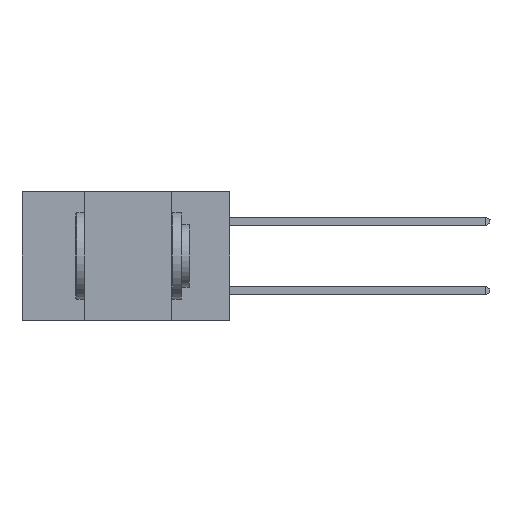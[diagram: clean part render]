
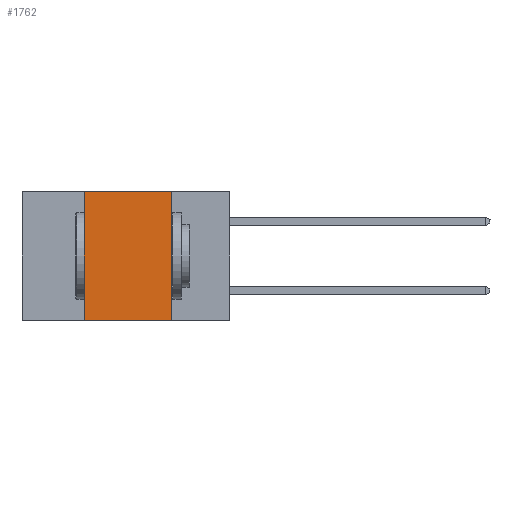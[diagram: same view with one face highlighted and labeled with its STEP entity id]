
A CAD part, left-side view. The second image highlights one B-rep face of the part: STEP entity #1762.
In plain terms, the highlighted planar face has unit normal (-1, 0, 0).
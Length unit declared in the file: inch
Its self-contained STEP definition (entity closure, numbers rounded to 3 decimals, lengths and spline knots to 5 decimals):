
#173 = CARTESIAN_POINT ( 'NONE',  ( 0., 0.6, 0. ) ) ;
#1762 = ADVANCED_FACE ( 'NONE', ( #4417 ), #4195, .F. ) ;
#1838 = CARTESIAN_POINT ( 'NONE',  ( 0., 0.42, -0.37 ) ) ;
#1903 = VECTOR ( 'NONE', #13524, 39.37008 ) ;
#2373 = EDGE_LOOP ( 'NONE', ( #3141, #16533, #15461, #11650 ) ) ;
#2623 = VECTOR ( 'NONE', #15800, 39.37008 ) ;
#3141 = ORIENTED_EDGE ( 'NONE', *, *, #5247, .F. ) ;
#3207 = CARTESIAN_POINT ( 'NONE',  ( 0., 0.17, -0.37 ) ) ;
#3596 = LINE ( 'NONE', #8348, #1903 ) ;
#4195 = PLANE ( 'NONE',  #13025 ) ;
#4417 = FACE_OUTER_BOUND ( 'NONE', #2373, .T. ) ;
#4685 = EDGE_CURVE ( 'NONE', #15388, #20979, #11557, .T. ) ;
#5247 = EDGE_CURVE ( 'NONE', #20444, #20979, #20769, .T. ) ;
#5276 = DIRECTION ( 'NONE',  ( 0., 0., -1. ) ) ;
#6138 = VECTOR ( 'NONE', #5276, 39.37008 ) ;
#7793 = DIRECTION ( 'NONE',  ( 0., 0., -1. ) ) ;
#8348 = CARTESIAN_POINT ( 'NONE',  ( 0., 0.42, -0.37 ) ) ;
#11557 = LINE ( 'NONE', #15543, #18306 ) ;
#11650 = ORIENTED_EDGE ( 'NONE', *, *, #4685, .T. ) ;
#12281 = EDGE_CURVE ( 'NONE', #21394, #20444, #15593, .T. ) ;
#12567 = EDGE_CURVE ( 'NONE', #15388, #21394, #3596, .T. ) ;
#13025 = AXIS2_PLACEMENT_3D ( 'NONE', #14749, #16338, #7793 ) ;
#13524 = DIRECTION ( 'NONE',  ( 0., 0., 1. ) ) ;
#14749 = CARTESIAN_POINT ( 'NONE',  ( 0., 0.6, 0. ) ) ;
#15388 = VERTEX_POINT ( 'NONE', #1838 ) ;
#15446 = CARTESIAN_POINT ( 'NONE',  ( 0., 0.42, 0. ) ) ;
#15461 = ORIENTED_EDGE ( 'NONE', *, *, #12567, .F. ) ;
#15543 = CARTESIAN_POINT ( 'NONE',  ( 0., 0.6, -0.37 ) ) ;
#15593 = LINE ( 'NONE', #173, #2623 ) ;
#15800 = DIRECTION ( 'NONE',  ( 0., -1., 0. ) ) ;
#16338 = DIRECTION ( 'NONE',  ( 1., 0., 0. ) ) ;
#16533 = ORIENTED_EDGE ( 'NONE', *, *, #12281, .F. ) ;
#16595 = DIRECTION ( 'NONE',  ( 0., -1., 0. ) ) ;
#18306 = VECTOR ( 'NONE', #16595, 39.37008 ) ;
#20444 = VERTEX_POINT ( 'NONE', #21460 ) ;
#20769 = LINE ( 'NONE', #20882, #6138 ) ;
#20882 = CARTESIAN_POINT ( 'NONE',  ( 0., 0.17, -0.37 ) ) ;
#20979 = VERTEX_POINT ( 'NONE', #3207 ) ;
#21394 = VERTEX_POINT ( 'NONE', #15446 ) ;
#21460 = CARTESIAN_POINT ( 'NONE',  ( 0., 0.17, 0. ) ) ;
